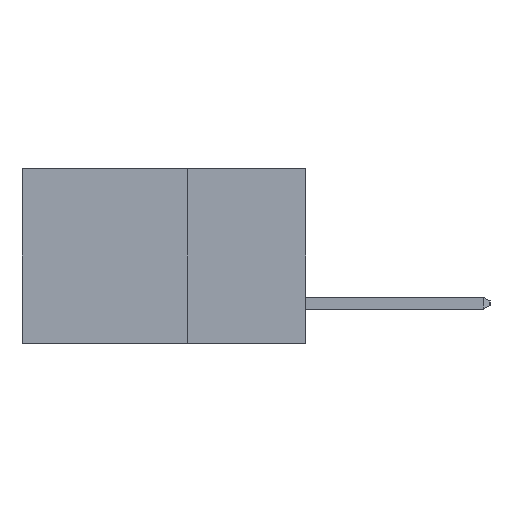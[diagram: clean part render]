
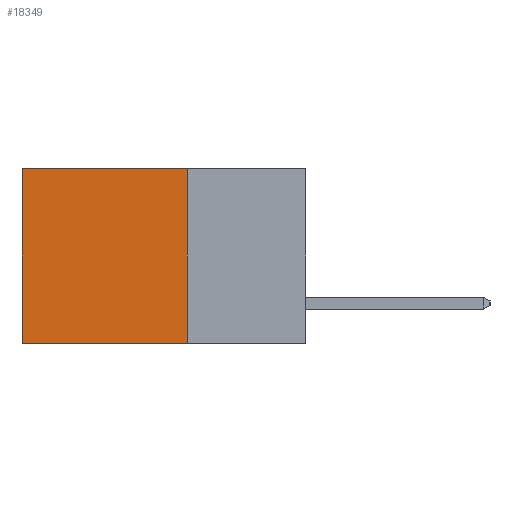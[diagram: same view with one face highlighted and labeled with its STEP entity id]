
A CAD part, left-side view. The second image highlights one B-rep face of the part: STEP entity #18349.
In plain terms, the highlighted planar face has unit normal (-1, 0, 0).
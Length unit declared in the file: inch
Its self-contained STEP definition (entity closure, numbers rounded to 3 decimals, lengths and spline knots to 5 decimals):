
#432 = DIRECTION ( 'NONE',  ( 0., 0., -1. ) ) ;
#771 = LINE ( 'NONE', #7760, #26429 ) ;
#965 = CARTESIAN_POINT ( 'NONE',  ( 0.298, 0.25, 0. ) ) ;
#1104 = LINE ( 'NONE', #16558, #20777 ) ;
#1515 = EDGE_CURVE ( 'NONE', #11682, #16462, #1104, .T. ) ;
#2813 = VERTEX_POINT ( 'NONE', #15022 ) ;
#4612 = CARTESIAN_POINT ( 'NONE',  ( 0.298, 0.6, 0. ) ) ;
#4932 = VECTOR ( 'NONE', #12642, 39.37008 ) ;
#5721 = ORIENTED_EDGE ( 'NONE', *, *, #18903, .T. ) ;
#6003 = CARTESIAN_POINT ( 'NONE',  ( 0.298, 0.25, 0. ) ) ;
#6443 = LINE ( 'NONE', #4612, #17034 ) ;
#6473 = CARTESIAN_POINT ( 'NONE',  ( 0.298, 0.25, -0.37 ) ) ;
#6675 = DIRECTION ( 'NONE',  ( 0., 0., -1. ) ) ;
#7674 = ORIENTED_EDGE ( 'NONE', *, *, #1515, .F. ) ;
#7760 = CARTESIAN_POINT ( 'NONE',  ( 0.298, 0.25, 0. ) ) ;
#8159 = DIRECTION ( 'NONE',  ( 1., 0., 0. ) ) ;
#9128 = FACE_OUTER_BOUND ( 'NONE', #25671, .T. ) ;
#10266 = AXIS2_PLACEMENT_3D ( 'NONE', #6003, #8159, #22617 ) ;
#10620 = LINE ( 'NONE', #16781, #4932 ) ;
#11072 = VERTEX_POINT ( 'NONE', #15962 ) ;
#11682 = VERTEX_POINT ( 'NONE', #965 ) ;
#12642 = DIRECTION ( 'NONE',  ( 0., 1., 0. ) ) ;
#15022 = CARTESIAN_POINT ( 'NONE',  ( 0.298, 0.6, -0.37 ) ) ;
#15734 = EDGE_CURVE ( 'NONE', #16462, #2813, #10620, .T. ) ;
#15962 = CARTESIAN_POINT ( 'NONE',  ( 0.298, 0.6, 0. ) ) ;
#16462 = VERTEX_POINT ( 'NONE', #6473 ) ;
#16558 = CARTESIAN_POINT ( 'NONE',  ( 0.298, 0.25, 0. ) ) ;
#16781 = CARTESIAN_POINT ( 'NONE',  ( 0.298, 0.25, -0.37 ) ) ;
#17034 = VECTOR ( 'NONE', #432, 39.37008 ) ;
#18349 = ADVANCED_FACE ( 'NONE', ( #9128 ), #20607, .F. ) ;
#18903 = EDGE_CURVE ( 'NONE', #11682, #11072, #771, .T. ) ;
#20607 = PLANE ( 'NONE',  #10266 ) ;
#20777 = VECTOR ( 'NONE', #6675, 39.37008 ) ;
#20858 = ORIENTED_EDGE ( 'NONE', *, *, #23015, .T. ) ;
#22243 = DIRECTION ( 'NONE',  ( 0., 1., 0. ) ) ;
#22617 = DIRECTION ( 'NONE',  ( 0., 0., -1. ) ) ;
#23015 = EDGE_CURVE ( 'NONE', #11072, #2813, #6443, .T. ) ;
#25653 = ORIENTED_EDGE ( 'NONE', *, *, #15734, .F. ) ;
#25671 = EDGE_LOOP ( 'NONE', ( #20858, #25653, #7674, #5721 ) ) ;
#26429 = VECTOR ( 'NONE', #22243, 39.37008 ) ;
